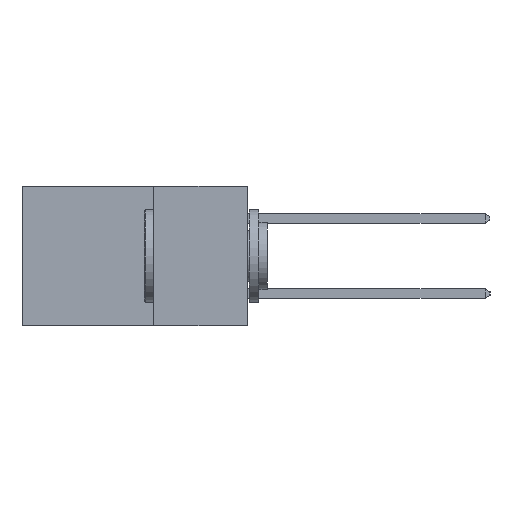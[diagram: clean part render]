
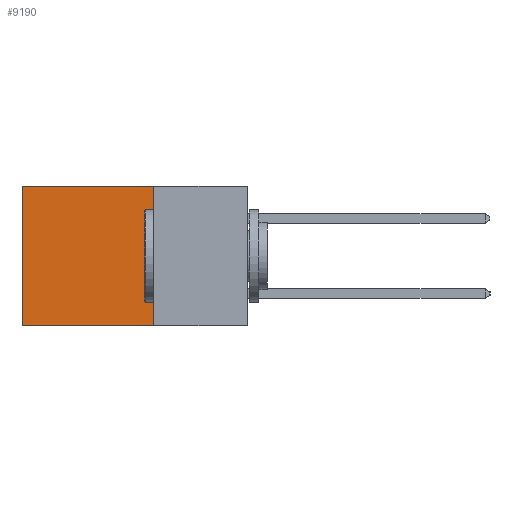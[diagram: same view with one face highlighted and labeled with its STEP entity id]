
A CAD part, left-side view. The second image highlights one B-rep face of the part: STEP entity #9190.
In plain terms, the highlighted planar face has unit normal (-1, 0, 0).
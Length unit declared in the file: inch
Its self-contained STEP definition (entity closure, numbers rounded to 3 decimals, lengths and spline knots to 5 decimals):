
#830 = FACE_OUTER_BOUND ( 'NONE', #17485, .T. ) ;
#1338 = ORIENTED_EDGE ( 'NONE', *, *, #7686, .T. ) ;
#1806 = CARTESIAN_POINT ( 'NONE',  ( 0.2615, 0.6, -0.37 ) ) ;
#2119 = LINE ( 'NONE', #5784, #10991 ) ;
#3095 = CARTESIAN_POINT ( 'NONE',  ( 0.2615, 0.25, -0.37 ) ) ;
#4026 = VECTOR ( 'NONE', #4760, 39.37008 ) ;
#4044 = ORIENTED_EDGE ( 'NONE', *, *, #17888, .T. ) ;
#4760 = DIRECTION ( 'NONE',  ( 0., 1., 0. ) ) ;
#5249 = VERTEX_POINT ( 'NONE', #17905 ) ;
#5784 = CARTESIAN_POINT ( 'NONE',  ( 0.2615, 0.25, 0. ) ) ;
#5825 = EDGE_CURVE ( 'NONE', #19351, #5249, #11921, .T. ) ;
#6242 = VERTEX_POINT ( 'NONE', #7252 ) ;
#7252 = CARTESIAN_POINT ( 'NONE',  ( 0.2615, 0.6, -0.37 ) ) ;
#7383 = CARTESIAN_POINT ( 'NONE',  ( 0.2615, 0.6, 0. ) ) ;
#7442 = VECTOR ( 'NONE', #11936, 39.37008 ) ;
#7686 = EDGE_CURVE ( 'NONE', #13055, #6242, #20713, .T. ) ;
#7920 = ORIENTED_EDGE ( 'NONE', *, *, #13893, .F. ) ;
#8050 = CARTESIAN_POINT ( 'NONE',  ( 0.2615, 0.25, -0.37 ) ) ;
#8960 = ORIENTED_EDGE ( 'NONE', *, *, #5825, .F. ) ;
#9190 = ADVANCED_FACE ( 'NONE', ( #830 ), #17663, .F. ) ;
#9705 = DIRECTION ( 'NONE',  ( 1., 0., 0. ) ) ;
#10991 = VECTOR ( 'NONE', #17116, 39.37008 ) ;
#11921 = LINE ( 'NONE', #15997, #15614 ) ;
#11936 = DIRECTION ( 'NONE',  ( 0., 0., -1. ) ) ;
#13055 = VERTEX_POINT ( 'NONE', #7383 ) ;
#13893 = EDGE_CURVE ( 'NONE', #5249, #6242, #17014, .T. ) ;
#14025 = AXIS2_PLACEMENT_3D ( 'NONE', #8050, #9705, #20822 ) ;
#15614 = VECTOR ( 'NONE', #15936, 39.37008 ) ;
#15936 = DIRECTION ( 'NONE',  ( 0., 0., -1. ) ) ;
#15997 = CARTESIAN_POINT ( 'NONE',  ( 0.2615, 0.25, -0.37 ) ) ;
#17014 = LINE ( 'NONE', #3095, #4026 ) ;
#17116 = DIRECTION ( 'NONE',  ( 0., 1., 0. ) ) ;
#17485 = EDGE_LOOP ( 'NONE', ( #1338, #7920, #8960, #4044 ) ) ;
#17663 = PLANE ( 'NONE',  #14025 ) ;
#17888 = EDGE_CURVE ( 'NONE', #19351, #13055, #2119, .T. ) ;
#17905 = CARTESIAN_POINT ( 'NONE',  ( 0.2615, 0.25, -0.37 ) ) ;
#18761 = CARTESIAN_POINT ( 'NONE',  ( 0.2615, 0.25, 0. ) ) ;
#19351 = VERTEX_POINT ( 'NONE', #18761 ) ;
#20713 = LINE ( 'NONE', #1806, #7442 ) ;
#20822 = DIRECTION ( 'NONE',  ( 0., 0., -1. ) ) ;
